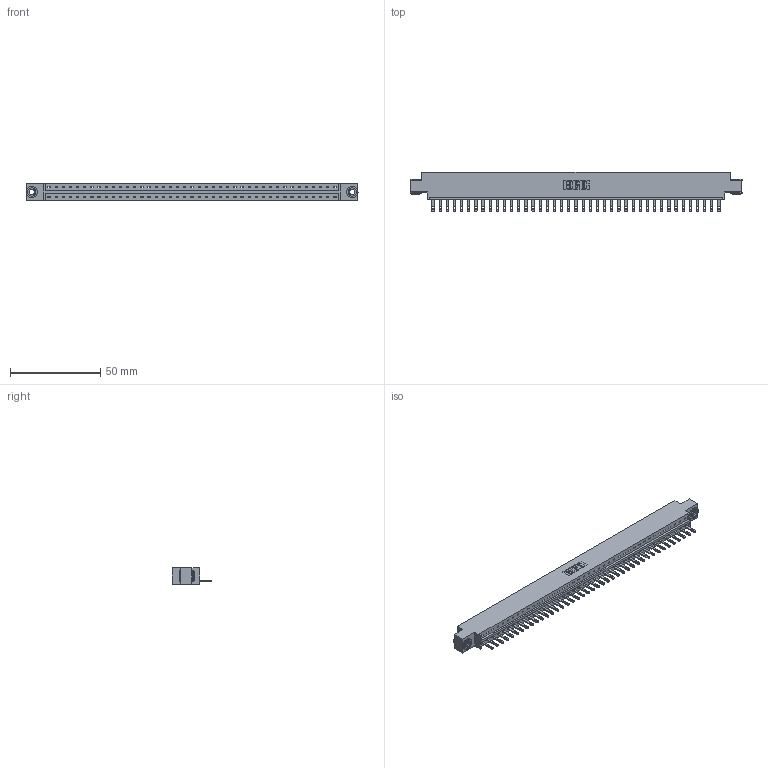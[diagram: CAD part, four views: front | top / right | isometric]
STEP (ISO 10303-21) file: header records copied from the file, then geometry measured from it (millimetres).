
FILE_DESCRIPTION (( 'STEP AP203' ), '1' );
FILE_NAME ('833-041-500-603.STEP', '2020-06-03T18:32:43', ( '' ), ( '' ), 'SwSTEP 2.0', 'SolidWorks 2020', '' );
FILE_SCHEMA (( 'CONFIG_CONTROL_DESIGN' ));
Length unit declared in the file: inch
Products named in the file (4): 833 Part_Offset - .156 Dia - TH; 345-250-002_345-250-002-102; 833-041-500-603; 345-292-001_345-293-100
Assembly tree (44 placements, depth 2):
  833-041-500-603
    833 Part_Offset - .156 Dia - TH
    345-292-001_345-293-100  x41
    345-250-002_345-250-002-102  x2
Bounding box: 184 x 21.85 x 9.4 mm (x, y, z)
Volume: 18323.7 mm3; surface area: 20344.6 mm2
Topology: 44 solids, 44 shells, 2370 faces, 7287 edges, 4854 vertices
Faces by surface type: plane 1560, cylinder 802, cone 8
Entity records: 25906 total; most frequent: CARTESIAN_POINT 4448, ORIENTED_EDGE 4418, DIRECTION 3789, EDGE_CURVE 2209, VECTOR 2053, LINE 2053, VERTEX_POINT 1470, AXIS2_PLACEMENT_3D 868
